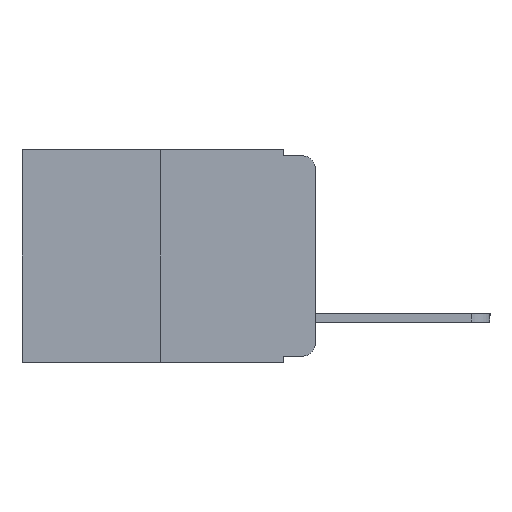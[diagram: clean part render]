
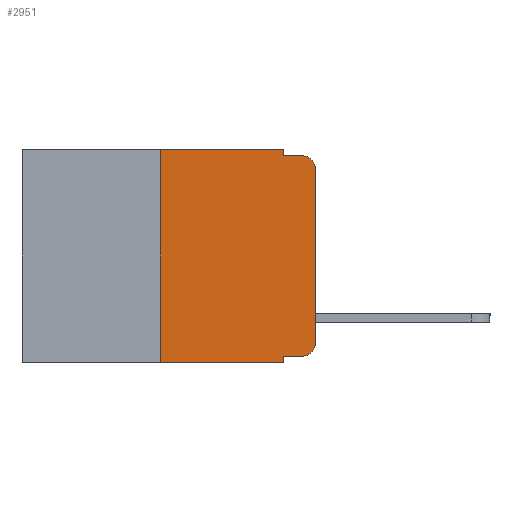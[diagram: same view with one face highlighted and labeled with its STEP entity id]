
A CAD part, left-side view. The second image highlights one B-rep face of the part: STEP entity #2951.
In plain terms, the highlighted planar face has unit normal (-1, 0, 0).
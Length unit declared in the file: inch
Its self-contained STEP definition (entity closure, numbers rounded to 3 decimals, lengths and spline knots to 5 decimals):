
#343 = CIRCLE ( 'NONE', #21383, 0.02 ) ;
#700 = LINE ( 'NONE', #8171, #4510 ) ;
#727 = EDGE_CURVE ( 'NONE', #19046, #17117, #3806, .T. ) ;
#1296 = EDGE_LOOP ( 'NONE', ( #19022, #4454, #5320, #6845, #18211, #3012, #3334, #7980, #4363, #15333 ) ) ;
#1971 = EDGE_CURVE ( 'NONE', #7699, #17117, #2574, .T. ) ;
#2047 = VERTEX_POINT ( 'NONE', #3780 ) ;
#2409 = CARTESIAN_POINT ( 'NONE',  ( 0., 0., -0.313 ) ) ;
#2429 = CARTESIAN_POINT ( 'NONE',  ( 0., 0.051, -0.333 ) ) ;
#2574 = CIRCLE ( 'NONE', #11387, 0.02 ) ;
#2951 = ADVANCED_FACE ( 'NONE', ( #10157 ), #5249, .F. ) ;
#3012 = ORIENTED_EDGE ( 'NONE', *, *, #20852, .F. ) ;
#3197 = VECTOR ( 'NONE', #22110, 39.37008 ) ;
#3224 = EDGE_CURVE ( 'NONE', #7608, #7699, #3700, .T. ) ;
#3245 = AXIS2_PLACEMENT_3D ( 'NONE', #15860, #15449, #15445 ) ;
#3334 = ORIENTED_EDGE ( 'NONE', *, *, #5136, .T. ) ;
#3700 = LINE ( 'NONE', #9835, #17783 ) ;
#3780 = CARTESIAN_POINT ( 'NONE',  ( 0., 0.02, -0.333 ) ) ;
#3806 = LINE ( 'NONE', #7178, #17891 ) ;
#4363 = ORIENTED_EDGE ( 'NONE', *, *, #18459, .T. ) ;
#4454 = ORIENTED_EDGE ( 'NONE', *, *, #1971, .T. ) ;
#4510 = VECTOR ( 'NONE', #10046, 39.37008 ) ;
#5136 = EDGE_CURVE ( 'NONE', #6541, #16861, #7168, .T. ) ;
#5249 = PLANE ( 'NONE',  #3245 ) ;
#5305 = CARTESIAN_POINT ( 'NONE',  ( 0., 0.473, -0.343 ) ) ;
#5320 = ORIENTED_EDGE ( 'NONE', *, *, #727, .F. ) ;
#5440 = EDGE_CURVE ( 'NONE', #13632, #6398, #700, .T. ) ;
#5449 = DIRECTION ( 'NONE',  ( 0., 0., 1. ) ) ;
#5752 = CARTESIAN_POINT ( 'NONE',  ( 0., 0.051, 0. ) ) ;
#6398 = VERTEX_POINT ( 'NONE', #5752 ) ;
#6523 = CARTESIAN_POINT ( 'NONE',  ( 0., 0., -0.03 ) ) ;
#6541 = VERTEX_POINT ( 'NONE', #17452 ) ;
#6586 = VECTOR ( 'NONE', #18050, 39.37008 ) ;
#6845 = ORIENTED_EDGE ( 'NONE', *, *, #22052, .F. ) ;
#6874 = CARTESIAN_POINT ( 'NONE',  ( 0., 0.051, -0.343 ) ) ;
#7168 = LINE ( 'NONE', #5305, #6586 ) ;
#7178 = CARTESIAN_POINT ( 'NONE',  ( 0., 0.051, -0.01 ) ) ;
#7608 = VERTEX_POINT ( 'NONE', #2409 ) ;
#7699 = VERTEX_POINT ( 'NONE', #6523 ) ;
#7980 = ORIENTED_EDGE ( 'NONE', *, *, #19652, .F. ) ;
#8043 = DIRECTION ( 'NONE',  ( 0., -1., 0. ) ) ;
#8171 = CARTESIAN_POINT ( 'NONE',  ( 0., 0.473, 0. ) ) ;
#8347 = VECTOR ( 'NONE', #5449, 39.37008 ) ;
#9835 = CARTESIAN_POINT ( 'NONE',  ( 0., 0., 0. ) ) ;
#9966 = DIRECTION ( 'NONE',  ( -1., 0., 0. ) ) ;
#10046 = DIRECTION ( 'NONE',  ( 0., -1., 0. ) ) ;
#10157 = FACE_OUTER_BOUND ( 'NONE', #1296, .T. ) ;
#11387 = AXIS2_PLACEMENT_3D ( 'NONE', #12864, #12813, #12784 ) ;
#11625 = LINE ( 'NONE', #16259, #14733 ) ;
#12544 = VERTEX_POINT ( 'NONE', #2429 ) ;
#12784 = DIRECTION ( 'NONE',  ( 0., 0., -1. ) ) ;
#12813 = DIRECTION ( 'NONE',  ( -1., 0., 0. ) ) ;
#12864 = CARTESIAN_POINT ( 'NONE',  ( 0., 0.02, -0.03 ) ) ;
#12983 = CARTESIAN_POINT ( 'NONE',  ( 0., 0.051, 0. ) ) ;
#13632 = VERTEX_POINT ( 'NONE', #14793 ) ;
#13745 = LINE ( 'NONE', #12983, #22685 ) ;
#14539 = DIRECTION ( 'NONE',  ( 0., 0., -1. ) ) ;
#14733 = VECTOR ( 'NONE', #14539, 39.37008 ) ;
#14793 = CARTESIAN_POINT ( 'NONE',  ( 0., 0.25, 0. ) ) ;
#14797 = DIRECTION ( 'NONE',  ( 0., 0., -1. ) ) ;
#15333 = ORIENTED_EDGE ( 'NONE', *, *, #17263, .T. ) ;
#15445 = DIRECTION ( 'NONE',  ( 0., 0., -1. ) ) ;
#15449 = DIRECTION ( 'NONE',  ( 1., 0., 0. ) ) ;
#15860 = CARTESIAN_POINT ( 'NONE',  ( 0., 0.473, 0. ) ) ;
#16259 = CARTESIAN_POINT ( 'NONE',  ( 0., 0.051, 0. ) ) ;
#16470 = CARTESIAN_POINT ( 'NONE',  ( 0., 0.25, 0. ) ) ;
#16703 = CARTESIAN_POINT ( 'NONE',  ( 0., 0.02, -0.01 ) ) ;
#16861 = VERTEX_POINT ( 'NONE', #6874 ) ;
#16895 = LINE ( 'NONE', #16470, #8347 ) ;
#17117 = VERTEX_POINT ( 'NONE', #16703 ) ;
#17263 = EDGE_CURVE ( 'NONE', #2047, #7608, #343, .T. ) ;
#17452 = CARTESIAN_POINT ( 'NONE',  ( 0., 0.25, -0.343 ) ) ;
#17783 = VECTOR ( 'NONE', #20325, 39.37008 ) ;
#17878 = LINE ( 'NONE', #20309, #3197 ) ;
#17891 = VECTOR ( 'NONE', #8043, 39.37008 ) ;
#18050 = DIRECTION ( 'NONE',  ( 0., -1., 0. ) ) ;
#18211 = ORIENTED_EDGE ( 'NONE', *, *, #5440, .F. ) ;
#18459 = EDGE_CURVE ( 'NONE', #12544, #2047, #17878, .T. ) ;
#19022 = ORIENTED_EDGE ( 'NONE', *, *, #3224, .T. ) ;
#19046 = VERTEX_POINT ( 'NONE', #22163 ) ;
#19652 = EDGE_CURVE ( 'NONE', #12544, #16861, #11625, .T. ) ;
#20309 = CARTESIAN_POINT ( 'NONE',  ( 0., 0.051, -0.333 ) ) ;
#20325 = DIRECTION ( 'NONE',  ( 0., 0., 1. ) ) ;
#20762 = CARTESIAN_POINT ( 'NONE',  ( 0., 0.02, -0.313 ) ) ;
#20852 = EDGE_CURVE ( 'NONE', #6541, #13632, #16895, .T. ) ;
#21383 = AXIS2_PLACEMENT_3D ( 'NONE', #20762, #9966, #22554 ) ;
#22052 = EDGE_CURVE ( 'NONE', #6398, #19046, #13745, .T. ) ;
#22110 = DIRECTION ( 'NONE',  ( 0., -1., 0. ) ) ;
#22163 = CARTESIAN_POINT ( 'NONE',  ( 0., 0.051, -0.01 ) ) ;
#22554 = DIRECTION ( 'NONE',  ( 0., 0., -1. ) ) ;
#22685 = VECTOR ( 'NONE', #14797, 39.37008 ) ;
